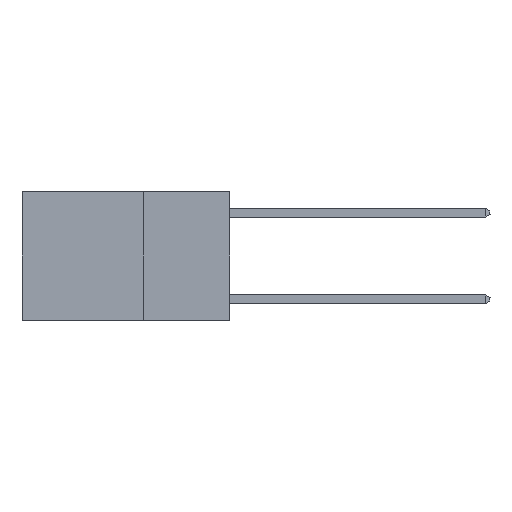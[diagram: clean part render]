
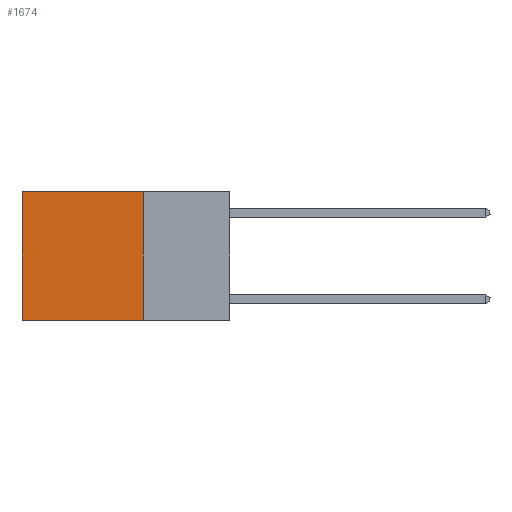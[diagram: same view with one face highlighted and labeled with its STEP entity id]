
A CAD part, left-side view. The second image highlights one B-rep face of the part: STEP entity #1674.
In plain terms, the highlighted planar face has unit normal (-1, 0, 0).
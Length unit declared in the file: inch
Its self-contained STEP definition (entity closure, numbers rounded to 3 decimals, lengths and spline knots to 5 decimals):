
#241 = CARTESIAN_POINT ( 'NONE',  ( 0.2625, 0.25, 0. ) ) ;
#500 = CARTESIAN_POINT ( 'NONE',  ( 0.2625, 0.6, 0. ) ) ;
#864 = CARTESIAN_POINT ( 'NONE',  ( 0.2625, 0.25, -0.37 ) ) ;
#1400 = CARTESIAN_POINT ( 'NONE',  ( 0.2625, 0.6, -0.37 ) ) ;
#1674 = ADVANCED_FACE ( 'NONE', ( #14447 ), #15926, .F. ) ;
#2908 = ORIENTED_EDGE ( 'NONE', *, *, #15790, .T. ) ;
#2958 = ORIENTED_EDGE ( 'NONE', *, *, #15079, .F. ) ;
#3753 = AXIS2_PLACEMENT_3D ( 'NONE', #16182, #16276, #4518 ) ;
#4027 = VERTEX_POINT ( 'NONE', #1400 ) ;
#4492 = DIRECTION ( 'NONE',  ( 0., 0., -1. ) ) ;
#4518 = DIRECTION ( 'NONE',  ( 0., 0., -1. ) ) ;
#5900 = CARTESIAN_POINT ( 'NONE',  ( 0.2625, 0.25, 0. ) ) ;
#5940 = EDGE_LOOP ( 'NONE', ( #2908, #15857, #2958, #10967 ) ) ;
#6476 = EDGE_CURVE ( 'NONE', #16407, #8906, #14766, .T. ) ;
#8289 = CARTESIAN_POINT ( 'NONE',  ( 0.2625, 0.6, 0. ) ) ;
#8444 = LINE ( 'NONE', #13614, #16233 ) ;
#8594 = CARTESIAN_POINT ( 'NONE',  ( 0.2625, 0.25, 0. ) ) ;
#8906 = VERTEX_POINT ( 'NONE', #8289 ) ;
#9680 = LINE ( 'NONE', #500, #16787 ) ;
#10967 = ORIENTED_EDGE ( 'NONE', *, *, #6476, .T. ) ;
#12402 = DIRECTION ( 'NONE',  ( 0., 1., 0. ) ) ;
#12634 = LINE ( 'NONE', #8594, #14840 ) ;
#13542 = DIRECTION ( 'NONE',  ( 0., 1., 0. ) ) ;
#13614 = CARTESIAN_POINT ( 'NONE',  ( 0.2625, 0.25, -0.37 ) ) ;
#14199 = VERTEX_POINT ( 'NONE', #864 ) ;
#14447 = FACE_OUTER_BOUND ( 'NONE', #5940, .T. ) ;
#14766 = LINE ( 'NONE', #241, #15472 ) ;
#14840 = VECTOR ( 'NONE', #16472, 39.37008 ) ;
#15079 = EDGE_CURVE ( 'NONE', #16407, #14199, #12634, .T. ) ;
#15472 = VECTOR ( 'NONE', #13542, 39.37008 ) ;
#15790 = EDGE_CURVE ( 'NONE', #8906, #4027, #9680, .T. ) ;
#15857 = ORIENTED_EDGE ( 'NONE', *, *, #15861, .F. ) ;
#15861 = EDGE_CURVE ( 'NONE', #14199, #4027, #8444, .T. ) ;
#15926 = PLANE ( 'NONE',  #3753 ) ;
#16182 = CARTESIAN_POINT ( 'NONE',  ( 0.2625, 0.25, 0. ) ) ;
#16233 = VECTOR ( 'NONE', #12402, 39.37008 ) ;
#16276 = DIRECTION ( 'NONE',  ( 1., 0., 0. ) ) ;
#16407 = VERTEX_POINT ( 'NONE', #5900 ) ;
#16472 = DIRECTION ( 'NONE',  ( 0., 0., -1. ) ) ;
#16787 = VECTOR ( 'NONE', #4492, 39.37008 ) ;
